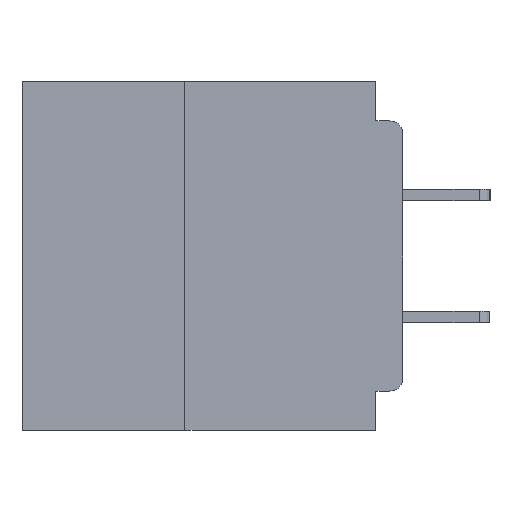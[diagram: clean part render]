
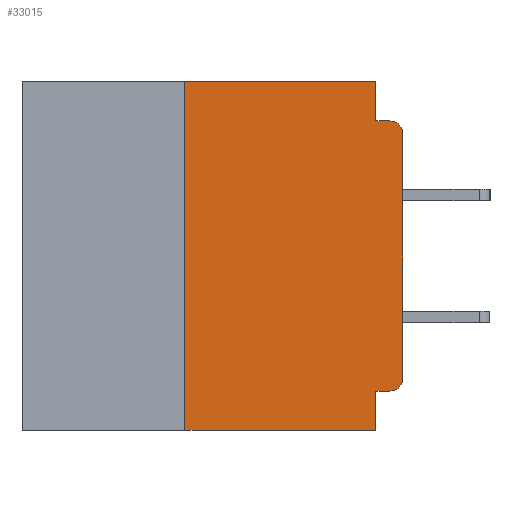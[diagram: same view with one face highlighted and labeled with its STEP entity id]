
A CAD part, left-side view. The second image highlights one B-rep face of the part: STEP entity #33015.
In plain terms, the highlighted planar face has unit normal (-1, 0, 0).
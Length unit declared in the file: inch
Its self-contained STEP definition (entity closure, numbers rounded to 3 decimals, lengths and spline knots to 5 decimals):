
#37 = EDGE_CURVE ( 'NONE', #21865, #1368, #32073, .T. ) ;
#1085 = ORIENTED_EDGE ( 'NONE', *, *, #13745, .F. ) ;
#1332 = CARTESIAN_POINT ( 'NONE',  ( 0., 0.031, 0. ) ) ;
#1368 = VERTEX_POINT ( 'NONE', #7040 ) ;
#1704 = CARTESIAN_POINT ( 'NONE',  ( 0., 0.031, 0. ) ) ;
#2199 = VERTEX_POINT ( 'NONE', #26603 ) ;
#2804 = VECTOR ( 'NONE', #18393, 39.37008 ) ;
#3501 = PLANE ( 'NONE',  #7873 ) ;
#3538 = LINE ( 'NONE', #14110, #26609 ) ;
#4263 = ORIENTED_EDGE ( 'NONE', *, *, #23386, .T. ) ;
#4365 = DIRECTION ( 'NONE',  ( 0., 0., 1. ) ) ;
#5124 = CARTESIAN_POINT ( 'NONE',  ( 0., 0.015, -0.355 ) ) ;
#5355 = CARTESIAN_POINT ( 'NONE',  ( 0., 0., -0.045 ) ) ;
#5946 = CARTESIAN_POINT ( 'NONE',  ( 0., 0.015, -0.045 ) ) ;
#5990 = VERTEX_POINT ( 'NONE', #17231 ) ;
#6401 = DIRECTION ( 'NONE',  ( 0., -1., 0. ) ) ;
#6780 = CARTESIAN_POINT ( 'NONE',  ( 0., 0.437, 0. ) ) ;
#7040 = CARTESIAN_POINT ( 'NONE',  ( 0., 0., -0.34 ) ) ;
#7348 = VERTEX_POINT ( 'NONE', #14107 ) ;
#7873 = AXIS2_PLACEMENT_3D ( 'NONE', #6780, #29721, #10080 ) ;
#8345 = DIRECTION ( 'NONE',  ( 0., -1., 0. ) ) ;
#8473 = CARTESIAN_POINT ( 'NONE',  ( 0., 0., -0.06 ) ) ;
#8852 = LINE ( 'NONE', #40601, #34990 ) ;
#9570 = LINE ( 'NONE', #1332, #35718 ) ;
#10080 = DIRECTION ( 'NONE',  ( 0., 0., -1. ) ) ;
#10429 = ORIENTED_EDGE ( 'NONE', *, *, #24259, .T. ) ;
#10653 = VERTEX_POINT ( 'NONE', #1704 ) ;
#12558 = VERTEX_POINT ( 'NONE', #8473 ) ;
#12869 = ORIENTED_EDGE ( 'NONE', *, *, #40853, .F. ) ;
#13480 = LINE ( 'NONE', #35768, #29895 ) ;
#13745 = EDGE_CURVE ( 'NONE', #2199, #5990, #3538, .T. ) ;
#13997 = CARTESIAN_POINT ( 'NONE',  ( 0., 0.031, -0.4 ) ) ;
#14029 = ORIENTED_EDGE ( 'NONE', *, *, #25219, .F. ) ;
#14107 = CARTESIAN_POINT ( 'NONE',  ( 0., 0.031, -0.045 ) ) ;
#14110 = CARTESIAN_POINT ( 'NONE',  ( 0., 0.25, -0.4 ) ) ;
#14765 = ORIENTED_EDGE ( 'NONE', *, *, #39616, .T. ) ;
#15690 = ORIENTED_EDGE ( 'NONE', *, *, #35813, .F. ) ;
#16065 = AXIS2_PLACEMENT_3D ( 'NONE', #18197, #41055, #21526 ) ;
#17053 = VECTOR ( 'NONE', #31598, 39.37008 ) ;
#17231 = CARTESIAN_POINT ( 'NONE',  ( 0., 0.25, 0. ) ) ;
#18197 = CARTESIAN_POINT ( 'NONE',  ( 0., 0.015, -0.06 ) ) ;
#18393 = DIRECTION ( 'NONE',  ( 0., 0., 1. ) ) ;
#18849 = VERTEX_POINT ( 'NONE', #23849 ) ;
#18938 = EDGE_CURVE ( 'NONE', #10653, #7348, #9570, .T. ) ;
#20888 = ORIENTED_EDGE ( 'NONE', *, *, #36773, .F. ) ;
#21062 = DIRECTION ( 'NONE',  ( 0., 0., -1. ) ) ;
#21293 = LINE ( 'NONE', #28135, #2804 ) ;
#21447 = DIRECTION ( 'NONE',  ( 0., 0., -1. ) ) ;
#21526 = DIRECTION ( 'NONE',  ( 0., 0., -1. ) ) ;
#21596 = DIRECTION ( 'NONE',  ( -1., 0., 0. ) ) ;
#21736 = CARTESIAN_POINT ( 'NONE',  ( 0., 0.015, -0.34 ) ) ;
#21865 = VERTEX_POINT ( 'NONE', #5124 ) ;
#22044 = ORIENTED_EDGE ( 'NONE', *, *, #37, .T. ) ;
#23386 = EDGE_CURVE ( 'NONE', #1368, #12558, #21293, .T. ) ;
#23849 = CARTESIAN_POINT ( 'NONE',  ( 0., 0.031, -0.355 ) ) ;
#24259 = EDGE_CURVE ( 'NONE', #2199, #38230, #13480, .T. ) ;
#24444 = CIRCLE ( 'NONE', #16065, 0.015 ) ;
#24795 = VERTEX_POINT ( 'NONE', #5946 ) ;
#25219 = EDGE_CURVE ( 'NONE', #5990, #10653, #36014, .T. ) ;
#25839 = FACE_OUTER_BOUND ( 'NONE', #35428, .T. ) ;
#26603 = CARTESIAN_POINT ( 'NONE',  ( 0., 0.25, -0.4 ) ) ;
#26609 = VECTOR ( 'NONE', #4365, 39.37008 ) ;
#27349 = VECTOR ( 'NONE', #8345, 39.37008 ) ;
#27570 = DIRECTION ( 'NONE',  ( 0., 0., -1. ) ) ;
#27845 = LINE ( 'NONE', #5355, #17053 ) ;
#28135 = CARTESIAN_POINT ( 'NONE',  ( 0., 0., 0. ) ) ;
#29721 = DIRECTION ( 'NONE',  ( 1., 0., 0. ) ) ;
#29895 = VECTOR ( 'NONE', #6401, 39.37008 ) ;
#30820 = VECTOR ( 'NONE', #38833, 39.37008 ) ;
#31261 = ORIENTED_EDGE ( 'NONE', *, *, #18938, .F. ) ;
#31598 = DIRECTION ( 'NONE',  ( 0., -1., 0. ) ) ;
#32073 = CIRCLE ( 'NONE', #37510, 0.015 ) ;
#32303 = CARTESIAN_POINT ( 'NONE',  ( 0., 0., -0.355 ) ) ;
#33015 = ADVANCED_FACE ( 'NONE', ( #25839 ), #3501, .F. ) ;
#34990 = VECTOR ( 'NONE', #21062, 39.37008 ) ;
#35428 = EDGE_LOOP ( 'NONE', ( #4263, #14765, #12869, #31261, #14029, #1085, #10429, #15690, #20888, #22044 ) ) ;
#35718 = VECTOR ( 'NONE', #27570, 39.37008 ) ;
#35768 = CARTESIAN_POINT ( 'NONE',  ( 0., 0.437, -0.4 ) ) ;
#35813 = EDGE_CURVE ( 'NONE', #18849, #38230, #8852, .T. ) ;
#36014 = LINE ( 'NONE', #40942, #27349 ) ;
#36773 = EDGE_CURVE ( 'NONE', #21865, #18849, #39467, .T. ) ;
#37510 = AXIS2_PLACEMENT_3D ( 'NONE', #21736, #21596, #21447 ) ;
#38230 = VERTEX_POINT ( 'NONE', #13997 ) ;
#38833 = DIRECTION ( 'NONE',  ( 0., 1., 0. ) ) ;
#39467 = LINE ( 'NONE', #32303, #30820 ) ;
#39616 = EDGE_CURVE ( 'NONE', #12558, #24795, #24444, .T. ) ;
#40601 = CARTESIAN_POINT ( 'NONE',  ( 0., 0.031, -0.4 ) ) ;
#40853 = EDGE_CURVE ( 'NONE', #7348, #24795, #27845, .T. ) ;
#40942 = CARTESIAN_POINT ( 'NONE',  ( 0., 0.437, 0. ) ) ;
#41055 = DIRECTION ( 'NONE',  ( -1., 0., 0. ) ) ;
